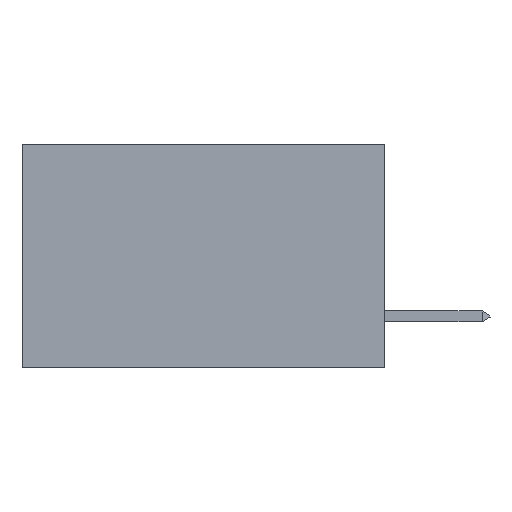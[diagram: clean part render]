
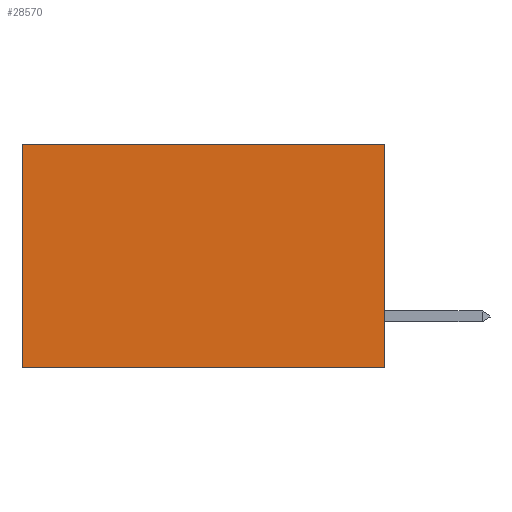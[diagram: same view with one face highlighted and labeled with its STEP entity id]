
A CAD part, left-side view. The second image highlights one B-rep face of the part: STEP entity #28570.
In plain terms, the highlighted planar face has unit normal (-1, 0, 0).
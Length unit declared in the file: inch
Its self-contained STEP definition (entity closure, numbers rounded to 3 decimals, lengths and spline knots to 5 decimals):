
#1422 = DIRECTION ( 'NONE',  ( 0., 1., 0. ) ) ;
#2221 = DIRECTION ( 'NONE',  ( 1., 0., 0. ) ) ;
#2904 = DIRECTION ( 'NONE',  ( 0., 0., -1. ) ) ;
#3141 = EDGE_LOOP ( 'NONE', ( #18675, #4306, #39436, #28953 ) ) ;
#3300 = VERTEX_POINT ( 'NONE', #37354 ) ;
#4306 = ORIENTED_EDGE ( 'NONE', *, *, #26262, .F. ) ;
#9421 = AXIS2_PLACEMENT_3D ( 'NONE', #21018, #2221, #2904 ) ;
#10639 = VERTEX_POINT ( 'NONE', #39613 ) ;
#11704 = CARTESIAN_POINT ( 'NONE',  ( 0.2875, 0., -0.37 ) ) ;
#11714 = LINE ( 'NONE', #28230, #35797 ) ;
#12823 = VERTEX_POINT ( 'NONE', #14941 ) ;
#13757 = DIRECTION ( 'NONE',  ( 0., 0., -1. ) ) ;
#14941 = CARTESIAN_POINT ( 'NONE',  ( 0.2875, 0.6, -0.37 ) ) ;
#17866 = PLANE ( 'NONE',  #9421 ) ;
#18675 = ORIENTED_EDGE ( 'NONE', *, *, #21897, .T. ) ;
#19456 = LINE ( 'NONE', #20194, #19953 ) ;
#19953 = VECTOR ( 'NONE', #1422, 39.37008 ) ;
#20194 = CARTESIAN_POINT ( 'NONE',  ( 0.2875, 0., -0.37 ) ) ;
#21018 = CARTESIAN_POINT ( 'NONE',  ( 0.2875, 0., 0. ) ) ;
#21897 = EDGE_CURVE ( 'NONE', #10639, #12823, #24342, .T. ) ;
#24342 = LINE ( 'NONE', #29583, #35620 ) ;
#25036 = DIRECTION ( 'NONE',  ( 0., 1., 0. ) ) ;
#26262 = EDGE_CURVE ( 'NONE', #27853, #12823, #19456, .T. ) ;
#27853 = VERTEX_POINT ( 'NONE', #11704 ) ;
#28116 = VECTOR ( 'NONE', #37671, 39.37008 ) ;
#28230 = CARTESIAN_POINT ( 'NONE',  ( 0.2875, 0., 0. ) ) ;
#28570 = ADVANCED_FACE ( 'NONE', ( #38520 ), #17866, .F. ) ;
#28953 = ORIENTED_EDGE ( 'NONE', *, *, #33258, .T. ) ;
#29583 = CARTESIAN_POINT ( 'NONE',  ( 0.2875, 0.6, 0. ) ) ;
#33258 = EDGE_CURVE ( 'NONE', #3300, #10639, #11714, .T. ) ;
#34361 = CARTESIAN_POINT ( 'NONE',  ( 0.2875, 0., 0. ) ) ;
#35620 = VECTOR ( 'NONE', #13757, 39.37008 ) ;
#35797 = VECTOR ( 'NONE', #25036, 39.37008 ) ;
#36781 = EDGE_CURVE ( 'NONE', #3300, #27853, #37921, .T. ) ;
#37354 = CARTESIAN_POINT ( 'NONE',  ( 0.2875, 0., 0. ) ) ;
#37671 = DIRECTION ( 'NONE',  ( 0., 0., -1. ) ) ;
#37921 = LINE ( 'NONE', #34361, #28116 ) ;
#38520 = FACE_OUTER_BOUND ( 'NONE', #3141, .T. ) ;
#39436 = ORIENTED_EDGE ( 'NONE', *, *, #36781, .F. ) ;
#39613 = CARTESIAN_POINT ( 'NONE',  ( 0.2875, 0.6, 0. ) ) ;
